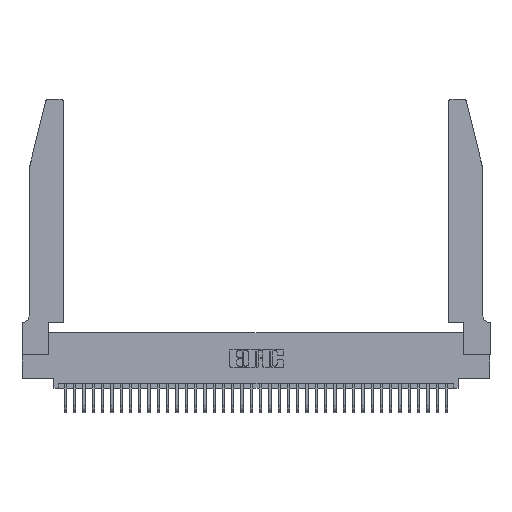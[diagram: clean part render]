
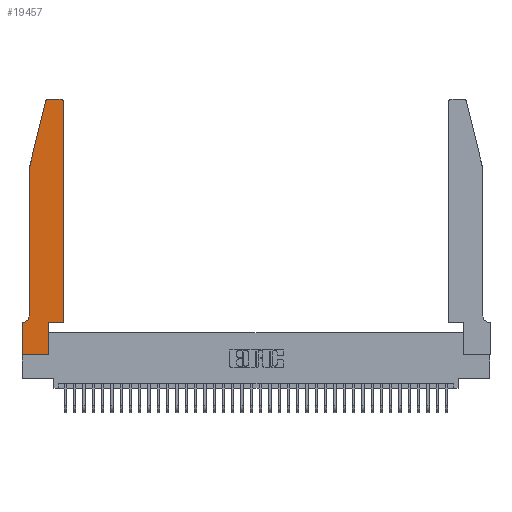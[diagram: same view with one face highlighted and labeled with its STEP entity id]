
A CAD part, top view. The second image highlights one B-rep face of the part: STEP entity #19457.
In plain terms, the highlighted planar face has unit normal (0, 0, 1).
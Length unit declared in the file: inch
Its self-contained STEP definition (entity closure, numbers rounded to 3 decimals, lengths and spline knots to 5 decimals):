
#10 = CARTESIAN_POINT ( 'NONE',  ( 0.0755, 2., 0.37 ) ) ;
#254 = LINE ( 'NONE', #27499, #7764 ) ;
#878 = ORIENTED_EDGE ( 'NONE', *, *, #36257, .T. ) ;
#1096 = VECTOR ( 'NONE', #29182, 39.37008 ) ;
#1158 = CARTESIAN_POINT ( 'NONE',  ( 0.4505, 0.35, 0.37 ) ) ;
#1180 = CARTESIAN_POINT ( 'NONE',  ( 0., 0.35, 0.37 ) ) ;
#2607 = EDGE_CURVE ( 'NONE', #12687, #21834, #26844, .T. ) ;
#2818 = EDGE_CURVE ( 'NONE', #15805, #31815, #33868, .T. ) ;
#2866 = ORIENTED_EDGE ( 'NONE', *, *, #2818, .T. ) ;
#2992 = CARTESIAN_POINT ( 'NONE',  ( 0.2865, 0.35, 0.37 ) ) ;
#3082 = CIRCLE ( 'NONE', #25035, 0.07 ) ;
#3365 = LINE ( 'NONE', #11221, #4228 ) ;
#4003 = DIRECTION ( 'NONE',  ( 1., 0., 0. ) ) ;
#4228 = VECTOR ( 'NONE', #30971, 39.37008 ) ;
#4304 = CIRCLE ( 'NONE', #32885, 0.03 ) ;
#4377 = DIRECTION ( 'NONE',  ( 0., 0., 1. ) ) ;
#4956 = LINE ( 'NONE', #19449, #26652 ) ;
#5797 = CARTESIAN_POINT ( 'NONE',  ( 0.0755, 2., 0.37 ) ) ;
#5885 = VECTOR ( 'NONE', #20036, 39.37008 ) ;
#6222 = LINE ( 'NONE', #27363, #34512 ) ;
#6320 = CARTESIAN_POINT ( 'NONE',  ( 0.2605, 2.75, 0.37 ) ) ;
#7004 = DIRECTION ( 'NONE',  ( 0., 0., 1. ) ) ;
#7077 = CARTESIAN_POINT ( 'NONE',  ( 0.4505, 2.72, 0.37 ) ) ;
#7350 = CARTESIAN_POINT ( 'NONE',  ( 0.25487, 2.72718, 0.37 ) ) ;
#7764 = VECTOR ( 'NONE', #30335, 39.37008 ) ;
#8001 = ORIENTED_EDGE ( 'NONE', *, *, #2607, .T. ) ;
#8326 = EDGE_CURVE ( 'NONE', #9657, #27752, #3082, .T. ) ;
#9192 = CARTESIAN_POINT ( 'NONE',  ( 0.4205, 2.75, 0.37 ) ) ;
#9257 = ORIENTED_EDGE ( 'NONE', *, *, #16688, .T. ) ;
#9657 = VERTEX_POINT ( 'NONE', #21782 ) ;
#10395 = AXIS2_PLACEMENT_3D ( 'NONE', #1180, #20966, #4003 ) ;
#10420 = EDGE_LOOP ( 'NONE', ( #878, #16818, #15088, #12222, #20231, #10995, #17336, #9257, #2866, #33723, #8001, #31972 ) ) ;
#10622 = CARTESIAN_POINT ( 'NONE',  ( 0.0055, 0.42, 0.37 ) ) ;
#10995 = ORIENTED_EDGE ( 'NONE', *, *, #23419, .T. ) ;
#11040 = DIRECTION ( 'NONE',  ( 0., -1., 0. ) ) ;
#11221 = CARTESIAN_POINT ( 'NONE',  ( 0.0755, 0.35, 0.37 ) ) ;
#11631 = EDGE_CURVE ( 'NONE', #24799, #28609, #21846, .T. ) ;
#12066 = FACE_OUTER_BOUND ( 'NONE', #10420, .T. ) ;
#12222 = ORIENTED_EDGE ( 'NONE', *, *, #34976, .T. ) ;
#12225 = VECTOR ( 'NONE', #34263, 39.37008 ) ;
#12687 = VERTEX_POINT ( 'NONE', #1158 ) ;
#12949 = CARTESIAN_POINT ( 'NONE',  ( 0.2865, 0., 0.37 ) ) ;
#13426 = CARTESIAN_POINT ( 'NONE',  ( 0., 0., 0.37 ) ) ;
#13487 = DIRECTION ( 'NONE',  ( -1., 0., 0. ) ) ;
#14871 = AXIS2_PLACEMENT_3D ( 'NONE', #21360, #4377, #24206 ) ;
#15088 = ORIENTED_EDGE ( 'NONE', *, *, #11631, .T. ) ;
#15588 = VERTEX_POINT ( 'NONE', #25942 ) ;
#15805 = VERTEX_POINT ( 'NONE', #12949 ) ;
#16333 = EDGE_CURVE ( 'NONE', #31815, #12687, #254, .T. ) ;
#16346 = VERTEX_POINT ( 'NONE', #13426 ) ;
#16688 = EDGE_CURVE ( 'NONE', #16346, #15805, #32003, .T. ) ;
#16818 = ORIENTED_EDGE ( 'NONE', *, *, #35894, .T. ) ;
#17336 = ORIENTED_EDGE ( 'NONE', *, *, #36523, .T. ) ;
#17388 = CARTESIAN_POINT ( 'NONE',  ( 0.2865, 0.35, 0.37 ) ) ;
#18102 = PLANE ( 'NONE',  #10395 ) ;
#18423 = VECTOR ( 'NONE', #24960, 39.37008 ) ;
#19449 = CARTESIAN_POINT ( 'NONE',  ( 0.0755, 2., 0.37 ) ) ;
#19457 = ADVANCED_FACE ( 'NONE', ( #12066 ), #18102, .T. ) ;
#20036 = DIRECTION ( 'NONE',  ( -0.239, -0.971, 0. ) ) ;
#20231 = ORIENTED_EDGE ( 'NONE', *, *, #8326, .T. ) ;
#20966 = DIRECTION ( 'NONE',  ( 0., 0., 1. ) ) ;
#21360 = CARTESIAN_POINT ( 'NONE',  ( 0.284, 2.72, 0.37 ) ) ;
#21372 = CARTESIAN_POINT ( 'NONE',  ( 0.284, 2.75, 0.37 ) ) ;
#21782 = CARTESIAN_POINT ( 'NONE',  ( 0.0755, 0.42, 0.37 ) ) ;
#21834 = VERTEX_POINT ( 'NONE', #7077 ) ;
#21846 = LINE ( 'NONE', #5797, #5885 ) ;
#22096 = CARTESIAN_POINT ( 'NONE',  ( 0.4505, 0.35, 0.37 ) ) ;
#23419 = EDGE_CURVE ( 'NONE', #27752, #15588, #3365, .T. ) ;
#23505 = CARTESIAN_POINT ( 'NONE',  ( 0., 0., 0.37 ) ) ;
#23980 = CARTESIAN_POINT ( 'NONE',  ( 0.4205, 2.72, 0.37 ) ) ;
#24206 = DIRECTION ( 'NONE',  ( 1., 0., 0. ) ) ;
#24435 = LINE ( 'NONE', #6320, #35846 ) ;
#24799 = VERTEX_POINT ( 'NONE', #7350 ) ;
#24960 = DIRECTION ( 'NONE',  ( 0., 1., 0. ) ) ;
#25035 = AXIS2_PLACEMENT_3D ( 'NONE', #10622, #30392, #13487 ) ;
#25942 = CARTESIAN_POINT ( 'NONE',  ( 0., 0.35, 0.37 ) ) ;
#26045 = VERTEX_POINT ( 'NONE', #21372 ) ;
#26649 = CIRCLE ( 'NONE', #14871, 0.03 ) ;
#26652 = VECTOR ( 'NONE', #11040, 39.37008 ) ;
#26818 = DIRECTION ( 'NONE',  ( 1., 0., 0. ) ) ;
#26844 = LINE ( 'NONE', #22096, #18423 ) ;
#27363 = CARTESIAN_POINT ( 'NONE',  ( 0., 0., 0.37 ) ) ;
#27499 = CARTESIAN_POINT ( 'NONE',  ( 0.4505, 0.35, 0.37 ) ) ;
#27752 = VERTEX_POINT ( 'NONE', #32891 ) ;
#28609 = VERTEX_POINT ( 'NONE', #10 ) ;
#28788 = EDGE_CURVE ( 'NONE', #21834, #36311, #4304, .T. ) ;
#29182 = DIRECTION ( 'NONE',  ( 1., 0., 0. ) ) ;
#30192 = DIRECTION ( 'NONE',  ( 0., -1., 0. ) ) ;
#30335 = DIRECTION ( 'NONE',  ( 1., 0., 0. ) ) ;
#30392 = DIRECTION ( 'NONE',  ( 0., 0., -1. ) ) ;
#30971 = DIRECTION ( 'NONE',  ( -1., 0., 0. ) ) ;
#31773 = DIRECTION ( 'NONE',  ( -1., 0., 0. ) ) ;
#31815 = VERTEX_POINT ( 'NONE', #2992 ) ;
#31972 = ORIENTED_EDGE ( 'NONE', *, *, #28788, .T. ) ;
#32003 = LINE ( 'NONE', #23505, #1096 ) ;
#32885 = AXIS2_PLACEMENT_3D ( 'NONE', #23980, #7004, #26818 ) ;
#32891 = CARTESIAN_POINT ( 'NONE',  ( 0.0055, 0.35, 0.37 ) ) ;
#33723 = ORIENTED_EDGE ( 'NONE', *, *, #16333, .T. ) ;
#33868 = LINE ( 'NONE', #17388, #12225 ) ;
#34263 = DIRECTION ( 'NONE',  ( 0., 1., 0. ) ) ;
#34512 = VECTOR ( 'NONE', #30192, 39.37008 ) ;
#34976 = EDGE_CURVE ( 'NONE', #28609, #9657, #4956, .T. ) ;
#35846 = VECTOR ( 'NONE', #31773, 39.37008 ) ;
#35894 = EDGE_CURVE ( 'NONE', #26045, #24799, #26649, .T. ) ;
#36257 = EDGE_CURVE ( 'NONE', #36311, #26045, #24435, .T. ) ;
#36311 = VERTEX_POINT ( 'NONE', #9192 ) ;
#36523 = EDGE_CURVE ( 'NONE', #15588, #16346, #6222, .T. ) ;
